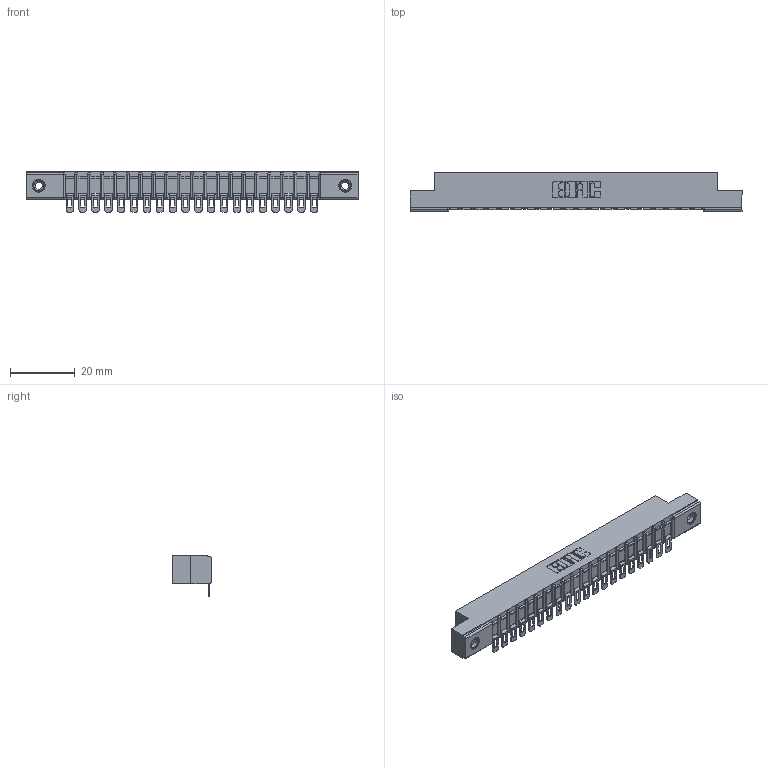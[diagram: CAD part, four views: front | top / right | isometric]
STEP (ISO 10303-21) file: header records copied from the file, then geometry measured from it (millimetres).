
FILE_DESCRIPTION (( 'STEP AP203' ), '1' );
FILE_NAME ('307-020-554-108.STEP', '2018-08-04T01:21:28', ( '' ), ( '' ), 'SwSTEP 2.0', 'SolidWorks 2016', '' );
FILE_SCHEMA (( 'CONFIG_CONTROL_DESIGN' ));
Length unit declared in the file: inch
Products named in the file (4): 307 Part_.156 Dia Mounting Holes; 307-290-002_554; 345-250-001_345-250-003-102; 307-020-554-108
Assembly tree (23 placements, depth 2):
  307-020-554-108
    307 Part_.156 Dia Mounting Holes
    307-290-002_554  x20
    345-250-001_345-250-003-102  x2
Bounding box: 102.26 x 12.01 x 12.52 mm (x, y, z)
Volume: 6750.7 mm3; surface area: 12268.1 mm2
Topology: 23 solids, 23 shells, 1819 faces, 5519 edges, 3614 vertices
Faces by surface type: plane 1022, cylinder 739, sphere 42, cone 12, torus 4
Entity records: 22008 total; most frequent: CARTESIAN_POINT 3689, ORIENTED_EDGE 3672, DIRECTION 3610, EDGE_CURVE 1836, VECTOR 1388, LINE 1388, VERTEX_POINT 1190, AXIS2_PLACEMENT_3D 1111
